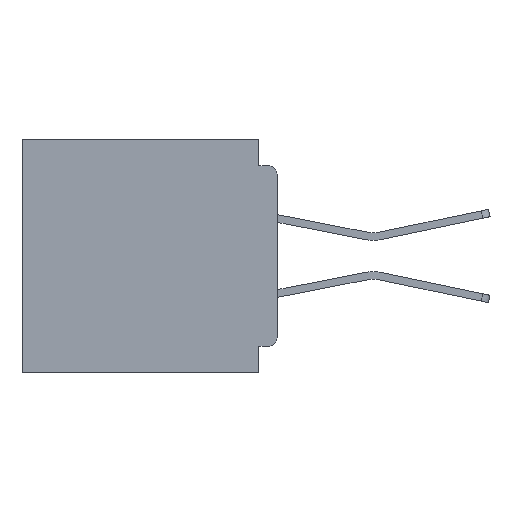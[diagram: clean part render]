
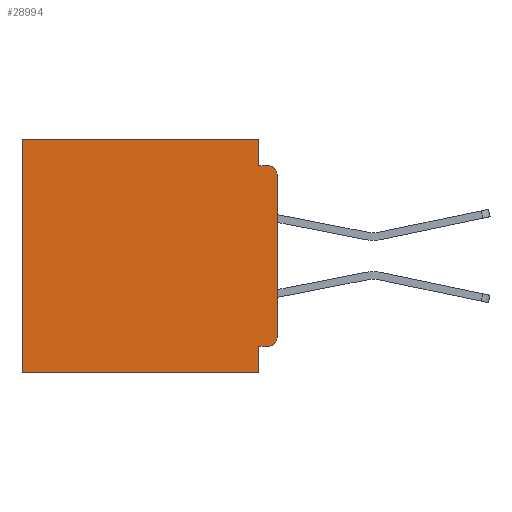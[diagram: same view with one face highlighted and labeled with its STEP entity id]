
A CAD part, left-side view. The second image highlights one B-rep face of the part: STEP entity #28994.
In plain terms, the highlighted planar face has unit normal (-1, 0, 0).
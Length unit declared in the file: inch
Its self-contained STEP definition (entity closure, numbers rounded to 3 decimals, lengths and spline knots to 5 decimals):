
#405 = VERTEX_POINT ( 'NONE', #36665 ) ;
#425 = DIRECTION ( 'NONE',  ( 0., 0., -1. ) ) ;
#844 = VECTOR ( 'NONE', #12574, 39.37008 ) ;
#926 = CARTESIAN_POINT ( 'NONE',  ( 0.3, 0., -0.4 ) ) ;
#2439 = VECTOR ( 'NONE', #23660, 39.37008 ) ;
#2780 = VECTOR ( 'NONE', #7765, 39.37008 ) ;
#3292 = ORIENTED_EDGE ( 'NONE', *, *, #33270, .F. ) ;
#3601 = CARTESIAN_POINT ( 'NONE',  ( 0.3, 0., 0. ) ) ;
#3775 = ORIENTED_EDGE ( 'NONE', *, *, #27529, .F. ) ;
#3822 = CARTESIAN_POINT ( 'NONE',  ( 0.3, 0., -0.355 ) ) ;
#4759 = CARTESIAN_POINT ( 'NONE',  ( 0.3, 0.015, -0.045 ) ) ;
#4945 = CARTESIAN_POINT ( 'NONE',  ( 0.3, 0., -0.4 ) ) ;
#5072 = VERTEX_POINT ( 'NONE', #7294 ) ;
#6328 = CIRCLE ( 'NONE', #23797, 0.015 ) ;
#6603 = DIRECTION ( 'NONE',  ( 0., 1., 0. ) ) ;
#6608 = AXIS2_PLACEMENT_3D ( 'NONE', #13648, #33636, #16508 ) ;
#6730 = ORIENTED_EDGE ( 'NONE', *, *, #30665, .T. ) ;
#7294 = CARTESIAN_POINT ( 'NONE',  ( 0.3, 0.031, -0.045 ) ) ;
#7765 = DIRECTION ( 'NONE',  ( 0., 1., 0. ) ) ;
#8979 = FACE_OUTER_BOUND ( 'NONE', #22497, .T. ) ;
#9222 = DIRECTION ( 'NONE',  ( 0., 1., 0. ) ) ;
#9741 = CARTESIAN_POINT ( 'NONE',  ( 0.3, 0.031, 0. ) ) ;
#10099 = LINE ( 'NONE', #3601, #16746 ) ;
#10313 = VERTEX_POINT ( 'NONE', #32423 ) ;
#11180 = ORIENTED_EDGE ( 'NONE', *, *, #29137, .F. ) ;
#11515 = DIRECTION ( 'NONE',  ( 0., 0., -1. ) ) ;
#11694 = LINE ( 'NONE', #27219, #33586 ) ;
#12092 = CARTESIAN_POINT ( 'NONE',  ( 0.3, 0., -0.06 ) ) ;
#12136 = VECTOR ( 'NONE', #6603, 39.37008 ) ;
#12509 = ORIENTED_EDGE ( 'NONE', *, *, #26300, .T. ) ;
#12574 = DIRECTION ( 'NONE',  ( 0., 0., -1. ) ) ;
#13413 = CIRCLE ( 'NONE', #6608, 0.015 ) ;
#13648 = CARTESIAN_POINT ( 'NONE',  ( 0.3, 0.015, -0.06 ) ) ;
#15680 = CARTESIAN_POINT ( 'NONE',  ( 0.3, 0.031, -0.4 ) ) ;
#15874 = LINE ( 'NONE', #9741, #844 ) ;
#16401 = VERTEX_POINT ( 'NONE', #4759 ) ;
#16508 = DIRECTION ( 'NONE',  ( 0., 0., -1. ) ) ;
#16648 = VERTEX_POINT ( 'NONE', #28524 ) ;
#16746 = VECTOR ( 'NONE', #9222, 39.37008 ) ;
#17345 = DIRECTION ( 'NONE',  ( -1., 0., 0. ) ) ;
#17692 = CARTESIAN_POINT ( 'NONE',  ( 0.3, 0., -0.045 ) ) ;
#17890 = EDGE_CURVE ( 'NONE', #405, #30618, #25447, .T. ) ;
#18565 = DIRECTION ( 'NONE',  ( 0., 0., -1. ) ) ;
#18820 = ORIENTED_EDGE ( 'NONE', *, *, #30836, .T. ) ;
#20606 = ORIENTED_EDGE ( 'NONE', *, *, #30112, .F. ) ;
#22497 = EDGE_LOOP ( 'NONE', ( #27210, #6730, #11180, #3292, #12509, #33553, #27764, #3775, #20606, #18820 ) ) ;
#22983 = VERTEX_POINT ( 'NONE', #26221 ) ;
#23660 = DIRECTION ( 'NONE',  ( 0., 0., -1. ) ) ;
#23797 = AXIS2_PLACEMENT_3D ( 'NONE', #34471, #17345, #425 ) ;
#24076 = AXIS2_PLACEMENT_3D ( 'NONE', #28529, #28641, #11515 ) ;
#24745 = VECTOR ( 'NONE', #18565, 39.37008 ) ;
#25447 = LINE ( 'NONE', #4945, #2780 ) ;
#25644 = LINE ( 'NONE', #15680, #24745 ) ;
#25790 = PLANE ( 'NONE',  #24076 ) ;
#26034 = CARTESIAN_POINT ( 'NONE',  ( 0.3, 0.437, -0.4 ) ) ;
#26221 = CARTESIAN_POINT ( 'NONE',  ( 0.3, 0., -0.34 ) ) ;
#26300 = EDGE_CURVE ( 'NONE', #10313, #16648, #10099, .T. ) ;
#27210 = ORIENTED_EDGE ( 'NONE', *, *, #28488, .F. ) ;
#27219 = CARTESIAN_POINT ( 'NONE',  ( 0.3, 0.437, -0.4 ) ) ;
#27529 = EDGE_CURVE ( 'NONE', #29383, #405, #25644, .T. ) ;
#27764 = ORIENTED_EDGE ( 'NONE', *, *, #17890, .F. ) ;
#28048 = CARTESIAN_POINT ( 'NONE',  ( 0.3, 0.015, -0.355 ) ) ;
#28076 = EDGE_CURVE ( 'NONE', #16648, #30618, #11694, .T. ) ;
#28488 = EDGE_CURVE ( 'NONE', #29610, #22983, #32658, .T. ) ;
#28524 = CARTESIAN_POINT ( 'NONE',  ( 0.3, 0.437, 0. ) ) ;
#28529 = CARTESIAN_POINT ( 'NONE',  ( 0.3, 0., -0.4 ) ) ;
#28641 = DIRECTION ( 'NONE',  ( 1., 0., 0. ) ) ;
#28994 = ADVANCED_FACE ( 'NONE', ( #8979 ), #25790, .F. ) ;
#29137 = EDGE_CURVE ( 'NONE', #5072, #16401, #33053, .T. ) ;
#29258 = DIRECTION ( 'NONE',  ( 0., -1., 0. ) ) ;
#29383 = VERTEX_POINT ( 'NONE', #30356 ) ;
#29610 = VERTEX_POINT ( 'NONE', #12092 ) ;
#30112 = EDGE_CURVE ( 'NONE', #30432, #29383, #34876, .T. ) ;
#30194 = DIRECTION ( 'NONE',  ( 0., 0., -1. ) ) ;
#30356 = CARTESIAN_POINT ( 'NONE',  ( 0.3, 0.031, -0.355 ) ) ;
#30432 = VERTEX_POINT ( 'NONE', #28048 ) ;
#30618 = VERTEX_POINT ( 'NONE', #26034 ) ;
#30665 = EDGE_CURVE ( 'NONE', #29610, #16401, #13413, .T. ) ;
#30836 = EDGE_CURVE ( 'NONE', #30432, #22983, #6328, .T. ) ;
#32171 = VECTOR ( 'NONE', #29258, 39.37008 ) ;
#32423 = CARTESIAN_POINT ( 'NONE',  ( 0.3, 0.031, 0. ) ) ;
#32658 = LINE ( 'NONE', #926, #2439 ) ;
#33053 = LINE ( 'NONE', #17692, #32171 ) ;
#33270 = EDGE_CURVE ( 'NONE', #10313, #5072, #15874, .T. ) ;
#33553 = ORIENTED_EDGE ( 'NONE', *, *, #28076, .T. ) ;
#33586 = VECTOR ( 'NONE', #30194, 39.37008 ) ;
#33636 = DIRECTION ( 'NONE',  ( -1., 0., 0. ) ) ;
#34471 = CARTESIAN_POINT ( 'NONE',  ( 0.3, 0.015, -0.34 ) ) ;
#34876 = LINE ( 'NONE', #3822, #12136 ) ;
#36665 = CARTESIAN_POINT ( 'NONE',  ( 0.3, 0.031, -0.4 ) ) ;
